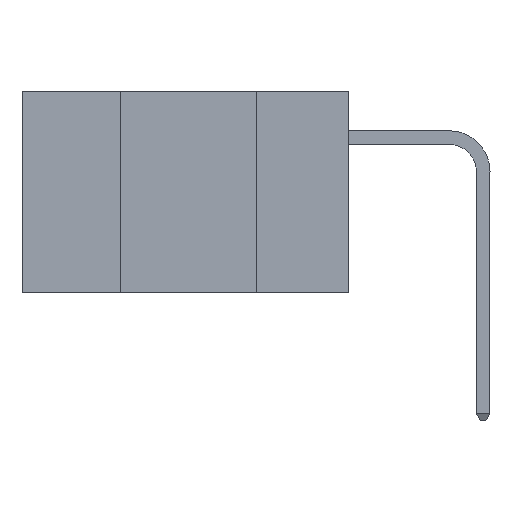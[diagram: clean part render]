
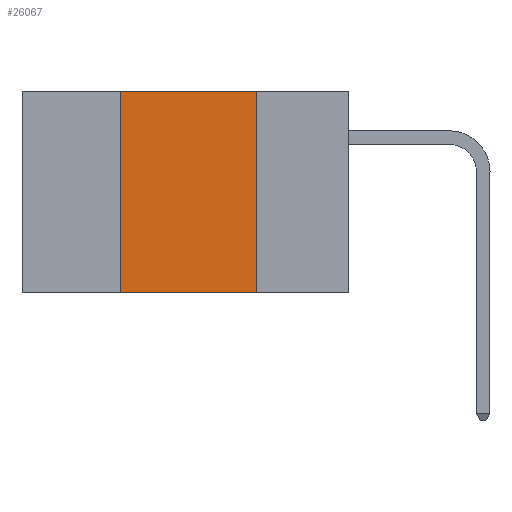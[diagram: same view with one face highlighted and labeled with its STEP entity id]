
A CAD part, left-side view. The second image highlights one B-rep face of the part: STEP entity #26067.
In plain terms, the highlighted planar face has unit normal (-1, 0, 0).
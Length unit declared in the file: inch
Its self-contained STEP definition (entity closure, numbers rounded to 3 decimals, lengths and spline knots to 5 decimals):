
#14 = FACE_OUTER_BOUND ( 'NONE', #7094, .T. ) ;
#494 = LINE ( 'NONE', #15143, #7462 ) ;
#512 = DIRECTION ( 'NONE',  ( 0., 0., -1. ) ) ;
#969 = DIRECTION ( 'NONE',  ( 1., 0., 0. ) ) ;
#1542 = CARTESIAN_POINT ( 'NONE',  ( 0., 0.42, 0. ) ) ;
#2679 = VECTOR ( 'NONE', #21145, 39.37008 ) ;
#3117 = CARTESIAN_POINT ( 'NONE',  ( 0., 0.17, -0.37 ) ) ;
#3670 = VERTEX_POINT ( 'NONE', #11450 ) ;
#4704 = LINE ( 'NONE', #25723, #26990 ) ;
#5419 = DIRECTION ( 'NONE',  ( 0., -1., 0. ) ) ;
#5460 = ORIENTED_EDGE ( 'NONE', *, *, #10054, .F. ) ;
#7094 = EDGE_LOOP ( 'NONE', ( #30858, #16420, #5460, #22731 ) ) ;
#7462 = VECTOR ( 'NONE', #512, 39.37008 ) ;
#10054 = EDGE_CURVE ( 'NONE', #10403, #35995, #18211, .T. ) ;
#10403 = VERTEX_POINT ( 'NONE', #31357 ) ;
#11236 = VERTEX_POINT ( 'NONE', #3117 ) ;
#11450 = CARTESIAN_POINT ( 'NONE',  ( 0., 0.17, 0. ) ) ;
#12491 = CARTESIAN_POINT ( 'NONE',  ( 0., 0.6, 0. ) ) ;
#12622 = PLANE ( 'NONE',  #30190 ) ;
#12912 = EDGE_CURVE ( 'NONE', #10403, #11236, #19456, .T. ) ;
#15143 = CARTESIAN_POINT ( 'NONE',  ( 0., 0.17, 0. ) ) ;
#16420 = ORIENTED_EDGE ( 'NONE', *, *, #25076, .F. ) ;
#18211 = LINE ( 'NONE', #18260, #2679 ) ;
#18260 = CARTESIAN_POINT ( 'NONE',  ( 0., 0.42, 0. ) ) ;
#19372 = DIRECTION ( 'NONE',  ( 0., -1., 0. ) ) ;
#19456 = LINE ( 'NONE', #25037, #25309 ) ;
#20449 = EDGE_CURVE ( 'NONE', #3670, #11236, #494, .T. ) ;
#21145 = DIRECTION ( 'NONE',  ( 0., 0., 1. ) ) ;
#21361 = DIRECTION ( 'NONE',  ( 0., 0., -1. ) ) ;
#22731 = ORIENTED_EDGE ( 'NONE', *, *, #12912, .T. ) ;
#25037 = CARTESIAN_POINT ( 'NONE',  ( 0., 0.6, -0.37 ) ) ;
#25076 = EDGE_CURVE ( 'NONE', #35995, #3670, #4704, .T. ) ;
#25309 = VECTOR ( 'NONE', #19372, 39.37008 ) ;
#25723 = CARTESIAN_POINT ( 'NONE',  ( 0., 0.6, 0. ) ) ;
#26067 = ADVANCED_FACE ( 'NONE', ( #14 ), #12622, .F. ) ;
#26990 = VECTOR ( 'NONE', #5419, 39.37008 ) ;
#30190 = AXIS2_PLACEMENT_3D ( 'NONE', #12491, #969, #21361 ) ;
#30858 = ORIENTED_EDGE ( 'NONE', *, *, #20449, .F. ) ;
#31357 = CARTESIAN_POINT ( 'NONE',  ( 0., 0.42, -0.37 ) ) ;
#35995 = VERTEX_POINT ( 'NONE', #1542 ) ;
